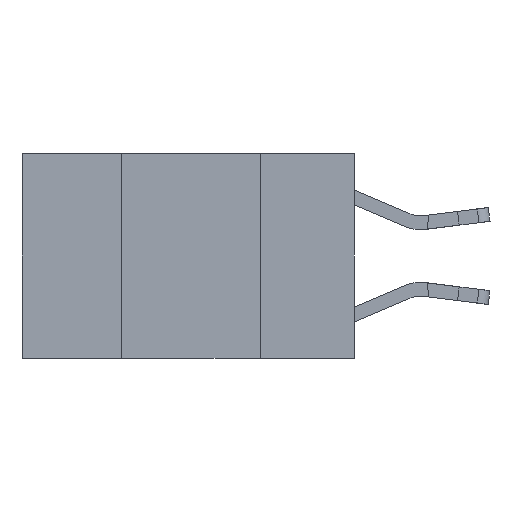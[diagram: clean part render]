
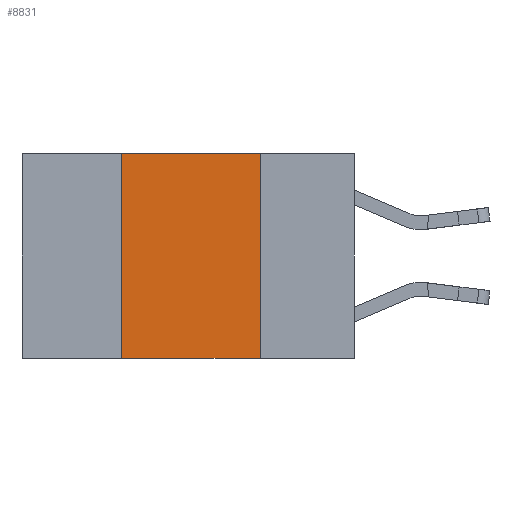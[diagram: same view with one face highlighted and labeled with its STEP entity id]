
A CAD part, left-side view. The second image highlights one B-rep face of the part: STEP entity #8831.
In plain terms, the highlighted planar face has unit normal (-1, 0, 0).
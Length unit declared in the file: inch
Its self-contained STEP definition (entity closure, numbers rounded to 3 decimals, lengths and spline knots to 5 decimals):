
#321 = CARTESIAN_POINT ( 'NONE',  ( 0., 0.42, 0. ) ) ;
#350 = CARTESIAN_POINT ( 'NONE',  ( 0., 0.42, 0. ) ) ;
#808 = FACE_OUTER_BOUND ( 'NONE', #4980, .T. ) ;
#1413 = CARTESIAN_POINT ( 'NONE',  ( 0., 0.17, 0. ) ) ;
#1451 = CARTESIAN_POINT ( 'NONE',  ( 0., 0.6, -0.37 ) ) ;
#1783 = VECTOR ( 'NONE', #5448, 39.37008 ) ;
#2122 = LINE ( 'NONE', #6032, #12629 ) ;
#2728 = EDGE_CURVE ( 'NONE', #7495, #7001, #9229, .T. ) ;
#2920 = CARTESIAN_POINT ( 'NONE',  ( 0., 0.6, 0. ) ) ;
#3700 = LINE ( 'NONE', #11373, #9600 ) ;
#3827 = DIRECTION ( 'NONE',  ( 0., 0., -1. ) ) ;
#3918 = LINE ( 'NONE', #321, #12040 ) ;
#4917 = ORIENTED_EDGE ( 'NONE', *, *, #6399, .F. ) ;
#4980 = EDGE_LOOP ( 'NONE', ( #4917, #6287, #5651, #7231 ) ) ;
#5448 = DIRECTION ( 'NONE',  ( 0., -1., 0. ) ) ;
#5651 = ORIENTED_EDGE ( 'NONE', *, *, #5820, .F. ) ;
#5820 = EDGE_CURVE ( 'NONE', #7495, #7790, #3918, .T. ) ;
#6017 = CARTESIAN_POINT ( 'NONE',  ( 0., 0.42, -0.37 ) ) ;
#6032 = CARTESIAN_POINT ( 'NONE',  ( 0., 0.6, 0. ) ) ;
#6095 = DIRECTION ( 'NONE',  ( 0., -1., 0. ) ) ;
#6287 = ORIENTED_EDGE ( 'NONE', *, *, #10139, .F. ) ;
#6399 = EDGE_CURVE ( 'NONE', #9888, #7001, #3700, .T. ) ;
#7001 = VERTEX_POINT ( 'NONE', #11599 ) ;
#7231 = ORIENTED_EDGE ( 'NONE', *, *, #2728, .T. ) ;
#7495 = VERTEX_POINT ( 'NONE', #6017 ) ;
#7651 = AXIS2_PLACEMENT_3D ( 'NONE', #2920, #8769, #3827 ) ;
#7790 = VERTEX_POINT ( 'NONE', #350 ) ;
#8769 = DIRECTION ( 'NONE',  ( 1., 0., 0. ) ) ;
#8831 = ADVANCED_FACE ( 'NONE', ( #808 ), #12703, .F. ) ;
#9229 = LINE ( 'NONE', #1451, #1783 ) ;
#9600 = VECTOR ( 'NONE', #12386, 39.37008 ) ;
#9888 = VERTEX_POINT ( 'NONE', #1413 ) ;
#10139 = EDGE_CURVE ( 'NONE', #7790, #9888, #2122, .T. ) ;
#11334 = DIRECTION ( 'NONE',  ( 0., 0., 1. ) ) ;
#11373 = CARTESIAN_POINT ( 'NONE',  ( 0., 0.17, 0. ) ) ;
#11599 = CARTESIAN_POINT ( 'NONE',  ( 0., 0.17, -0.37 ) ) ;
#12040 = VECTOR ( 'NONE', #11334, 39.37008 ) ;
#12386 = DIRECTION ( 'NONE',  ( 0., 0., -1. ) ) ;
#12629 = VECTOR ( 'NONE', #6095, 39.37008 ) ;
#12703 = PLANE ( 'NONE',  #7651 ) ;
